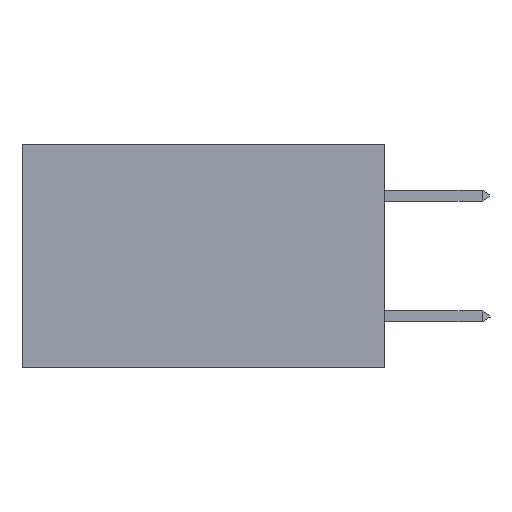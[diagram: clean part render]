
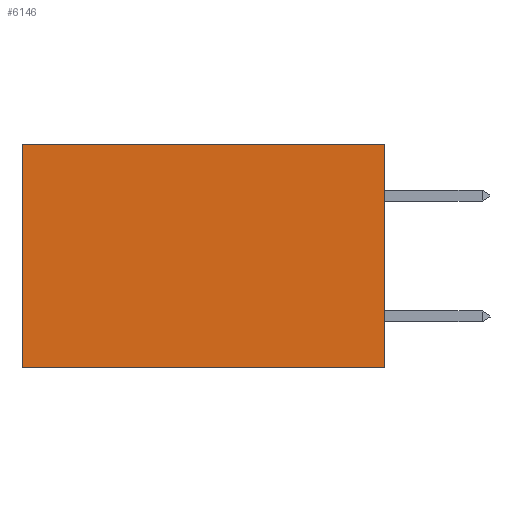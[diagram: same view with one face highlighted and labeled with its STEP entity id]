
A CAD part, left-side view. The second image highlights one B-rep face of the part: STEP entity #6146.
In plain terms, the highlighted planar face has unit normal (-1, 0, 0).
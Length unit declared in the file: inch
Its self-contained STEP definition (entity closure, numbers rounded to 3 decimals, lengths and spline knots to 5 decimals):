
#633 = CARTESIAN_POINT ( 'NONE',  ( 0.2875, 0., -0.37 ) ) ;
#931 = EDGE_LOOP ( 'NONE', ( #7062, #10059, #5932, #3526 ) ) ;
#994 = LINE ( 'NONE', #9758, #5967 ) ;
#1075 = VERTEX_POINT ( 'NONE', #5145 ) ;
#1345 = AXIS2_PLACEMENT_3D ( 'NONE', #6731, #10601, #10587 ) ;
#1724 = DIRECTION ( 'NONE',  ( 0., 1., 0. ) ) ;
#2502 = VECTOR ( 'NONE', #1724, 39.37008 ) ;
#2630 = CARTESIAN_POINT ( 'NONE',  ( 0.2875, 0., 0. ) ) ;
#3074 = PLANE ( 'NONE',  #1345 ) ;
#3385 = VERTEX_POINT ( 'NONE', #9969 ) ;
#3515 = DIRECTION ( 'NONE',  ( 0., 1., 0. ) ) ;
#3526 = ORIENTED_EDGE ( 'NONE', *, *, #7604, .T. ) ;
#3621 = EDGE_CURVE ( 'NONE', #3385, #1075, #7007, .T. ) ;
#4001 = CARTESIAN_POINT ( 'NONE',  ( 0.2875, 0., 0. ) ) ;
#4547 = EDGE_CURVE ( 'NONE', #8077, #3385, #10116, .T. ) ;
#5145 = CARTESIAN_POINT ( 'NONE',  ( 0.2875, 0.6, -0.37 ) ) ;
#5552 = FACE_OUTER_BOUND ( 'NONE', #931, .T. ) ;
#5658 = LINE ( 'NONE', #2630, #5926 ) ;
#5926 = VECTOR ( 'NONE', #3515, 39.37008 ) ;
#5932 = ORIENTED_EDGE ( 'NONE', *, *, #4547, .F. ) ;
#5950 = EDGE_CURVE ( 'NONE', #7137, #1075, #994, .T. ) ;
#5967 = VECTOR ( 'NONE', #9086, 39.37008 ) ;
#6146 = ADVANCED_FACE ( 'NONE', ( #5552 ), #3074, .F. ) ;
#6480 = CARTESIAN_POINT ( 'NONE',  ( 0.2875, 0.6, 0. ) ) ;
#6731 = CARTESIAN_POINT ( 'NONE',  ( 0.2875, 0., 0. ) ) ;
#7007 = LINE ( 'NONE', #633, #2502 ) ;
#7062 = ORIENTED_EDGE ( 'NONE', *, *, #5950, .T. ) ;
#7137 = VERTEX_POINT ( 'NONE', #6480 ) ;
#7604 = EDGE_CURVE ( 'NONE', #8077, #7137, #5658, .T. ) ;
#8077 = VERTEX_POINT ( 'NONE', #4001 ) ;
#8194 = VECTOR ( 'NONE', #9553, 39.37008 ) ;
#9086 = DIRECTION ( 'NONE',  ( 0., 0., -1. ) ) ;
#9553 = DIRECTION ( 'NONE',  ( 0., 0., -1. ) ) ;
#9758 = CARTESIAN_POINT ( 'NONE',  ( 0.2875, 0.6, 0. ) ) ;
#9969 = CARTESIAN_POINT ( 'NONE',  ( 0.2875, 0., -0.37 ) ) ;
#10059 = ORIENTED_EDGE ( 'NONE', *, *, #3621, .F. ) ;
#10116 = LINE ( 'NONE', #10491, #8194 ) ;
#10491 = CARTESIAN_POINT ( 'NONE',  ( 0.2875, 0., 0. ) ) ;
#10587 = DIRECTION ( 'NONE',  ( 0., 0., -1. ) ) ;
#10601 = DIRECTION ( 'NONE',  ( 1., 0., 0. ) ) ;
